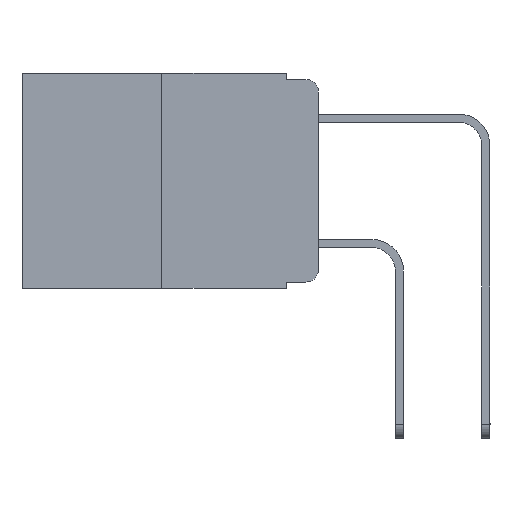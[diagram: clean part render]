
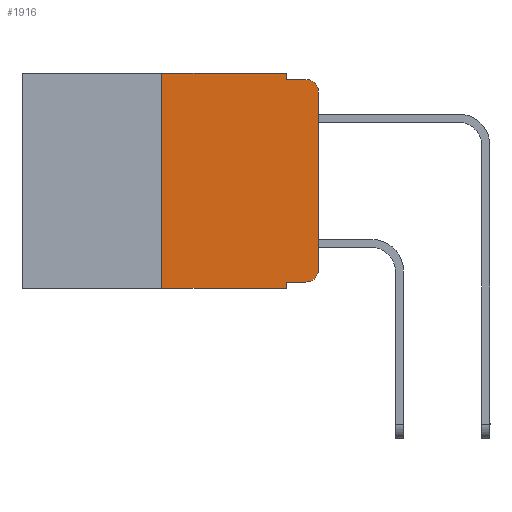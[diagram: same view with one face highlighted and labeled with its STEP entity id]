
A CAD part, left-side view. The second image highlights one B-rep face of the part: STEP entity #1916.
In plain terms, the highlighted planar face has unit normal (-1, 0, 0).
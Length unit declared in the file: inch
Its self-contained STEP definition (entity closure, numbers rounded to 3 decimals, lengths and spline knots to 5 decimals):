
#160 = VERTEX_POINT ( 'NONE', #13868 ) ;
#491 = EDGE_CURVE ( 'NONE', #12498, #5648, #8202, .T. ) ;
#499 = LINE ( 'NONE', #6336, #1512 ) ;
#860 = DIRECTION ( 'NONE',  ( 1., 0., 0. ) ) ;
#1202 = DIRECTION ( 'NONE',  ( 0., 0., -1. ) ) ;
#1274 = ORIENTED_EDGE ( 'NONE', *, *, #491, .F. ) ;
#1296 = CARTESIAN_POINT ( 'NONE',  ( 0., 0.051, 0. ) ) ;
#1490 = CARTESIAN_POINT ( 'NONE',  ( 0., 0.051, -0.01 ) ) ;
#1512 = VECTOR ( 'NONE', #4914, 39.37008 ) ;
#1516 = LINE ( 'NONE', #2947, #3714 ) ;
#1840 = LINE ( 'NONE', #9110, #1957 ) ;
#1916 = ADVANCED_FACE ( 'NONE', ( #6695 ), #9844, .F. ) ;
#1957 = VECTOR ( 'NONE', #5867, 39.37008 ) ;
#1971 = EDGE_CURVE ( 'NONE', #13129, #5648, #1516, .T. ) ;
#2947 = CARTESIAN_POINT ( 'NONE',  ( 0., 0.473, -0.343 ) ) ;
#2982 = AXIS2_PLACEMENT_3D ( 'NONE', #10653, #4445, #17731 ) ;
#3160 = DIRECTION ( 'NONE',  ( 0., 0., 1. ) ) ;
#3306 = DIRECTION ( 'NONE',  ( 0., -1., 0. ) ) ;
#3574 = EDGE_CURVE ( 'NONE', #14507, #5281, #10289, .T. ) ;
#3714 = VECTOR ( 'NONE', #8781, 39.37008 ) ;
#3920 = ORIENTED_EDGE ( 'NONE', *, *, #17124, .F. ) ;
#4060 = ORIENTED_EDGE ( 'NONE', *, *, #8865, .T. ) ;
#4135 = CARTESIAN_POINT ( 'NONE',  ( 0., 0.051, -0.343 ) ) ;
#4158 = CARTESIAN_POINT ( 'NONE',  ( 0., 0.051, 0. ) ) ;
#4445 = DIRECTION ( 'NONE',  ( -1., 0., 0. ) ) ;
#4520 = VERTEX_POINT ( 'NONE', #9346 ) ;
#4595 = ORIENTED_EDGE ( 'NONE', *, *, #5856, .F. ) ;
#4914 = DIRECTION ( 'NONE',  ( 0., -1., 0. ) ) ;
#5141 = AXIS2_PLACEMENT_3D ( 'NONE', #14288, #17167, #1202 ) ;
#5155 = EDGE_CURVE ( 'NONE', #13045, #14507, #5506, .T. ) ;
#5238 = EDGE_CURVE ( 'NONE', #4520, #13701, #1840, .T. ) ;
#5281 = VERTEX_POINT ( 'NONE', #14937 ) ;
#5506 = LINE ( 'NONE', #4158, #6525 ) ;
#5648 = VERTEX_POINT ( 'NONE', #4135 ) ;
#5746 = CIRCLE ( 'NONE', #2982, 0.02 ) ;
#5856 = EDGE_CURVE ( 'NONE', #13129, #7714, #10431, .T. ) ;
#5867 = DIRECTION ( 'NONE',  ( 0., 0., 1. ) ) ;
#6161 = ORIENTED_EDGE ( 'NONE', *, *, #5155, .F. ) ;
#6336 = CARTESIAN_POINT ( 'NONE',  ( 0., 0.051, -0.333 ) ) ;
#6525 = VECTOR ( 'NONE', #13028, 39.37008 ) ;
#6555 = DIRECTION ( 'NONE',  ( 0., -1., 0. ) ) ;
#6695 = FACE_OUTER_BOUND ( 'NONE', #8675, .T. ) ;
#7313 = CARTESIAN_POINT ( 'NONE',  ( 0., 0.25, 0. ) ) ;
#7714 = VERTEX_POINT ( 'NONE', #7313 ) ;
#8202 = LINE ( 'NONE', #1296, #11193 ) ;
#8411 = ORIENTED_EDGE ( 'NONE', *, *, #5238, .T. ) ;
#8675 = EDGE_LOOP ( 'NONE', ( #8411, #4060, #17378, #6161, #3920, #4595, #16260, #1274, #12161, #18448 ) ) ;
#8781 = DIRECTION ( 'NONE',  ( 0., -1., 0. ) ) ;
#8865 = EDGE_CURVE ( 'NONE', #13701, #5281, #16109, .T. ) ;
#8971 = EDGE_CURVE ( 'NONE', #160, #4520, #5746, .T. ) ;
#9110 = CARTESIAN_POINT ( 'NONE',  ( 0., 0., 0. ) ) ;
#9346 = CARTESIAN_POINT ( 'NONE',  ( 0., 0., -0.313 ) ) ;
#9844 = PLANE ( 'NONE',  #14367 ) ;
#10156 = VECTOR ( 'NONE', #3306, 39.37008 ) ;
#10289 = LINE ( 'NONE', #1490, #10156 ) ;
#10431 = LINE ( 'NONE', #16251, #10482 ) ;
#10482 = VECTOR ( 'NONE', #3160, 39.37008 ) ;
#10653 = CARTESIAN_POINT ( 'NONE',  ( 0., 0.02, -0.313 ) ) ;
#11193 = VECTOR ( 'NONE', #15460, 39.37008 ) ;
#11603 = CARTESIAN_POINT ( 'NONE',  ( 0., 0.051, 0. ) ) ;
#12161 = ORIENTED_EDGE ( 'NONE', *, *, #12189, .T. ) ;
#12189 = EDGE_CURVE ( 'NONE', #12498, #160, #499, .T. ) ;
#12429 = CARTESIAN_POINT ( 'NONE',  ( 0., 0.051, -0.333 ) ) ;
#12498 = VERTEX_POINT ( 'NONE', #12429 ) ;
#12514 = DIRECTION ( 'NONE',  ( 0., 0., -1. ) ) ;
#13028 = DIRECTION ( 'NONE',  ( 0., 0., -1. ) ) ;
#13045 = VERTEX_POINT ( 'NONE', #11603 ) ;
#13129 = VERTEX_POINT ( 'NONE', #15819 ) ;
#13337 = CARTESIAN_POINT ( 'NONE',  ( 0., 0.051, -0.01 ) ) ;
#13701 = VERTEX_POINT ( 'NONE', #17512 ) ;
#13868 = CARTESIAN_POINT ( 'NONE',  ( 0., 0.02, -0.333 ) ) ;
#14288 = CARTESIAN_POINT ( 'NONE',  ( 0., 0.02, -0.03 ) ) ;
#14367 = AXIS2_PLACEMENT_3D ( 'NONE', #15670, #860, #12514 ) ;
#14507 = VERTEX_POINT ( 'NONE', #13337 ) ;
#14937 = CARTESIAN_POINT ( 'NONE',  ( 0., 0.02, -0.01 ) ) ;
#15345 = LINE ( 'NONE', #18509, #16670 ) ;
#15460 = DIRECTION ( 'NONE',  ( 0., 0., -1. ) ) ;
#15670 = CARTESIAN_POINT ( 'NONE',  ( 0., 0.473, 0. ) ) ;
#15819 = CARTESIAN_POINT ( 'NONE',  ( 0., 0.25, -0.343 ) ) ;
#16109 = CIRCLE ( 'NONE', #5141, 0.02 ) ;
#16251 = CARTESIAN_POINT ( 'NONE',  ( 0., 0.25, 0. ) ) ;
#16260 = ORIENTED_EDGE ( 'NONE', *, *, #1971, .T. ) ;
#16670 = VECTOR ( 'NONE', #6555, 39.37008 ) ;
#17124 = EDGE_CURVE ( 'NONE', #7714, #13045, #15345, .T. ) ;
#17167 = DIRECTION ( 'NONE',  ( -1., 0., 0. ) ) ;
#17378 = ORIENTED_EDGE ( 'NONE', *, *, #3574, .F. ) ;
#17512 = CARTESIAN_POINT ( 'NONE',  ( 0., 0., -0.03 ) ) ;
#17731 = DIRECTION ( 'NONE',  ( 0., 0., -1. ) ) ;
#18448 = ORIENTED_EDGE ( 'NONE', *, *, #8971, .T. ) ;
#18509 = CARTESIAN_POINT ( 'NONE',  ( 0., 0.473, 0. ) ) ;
